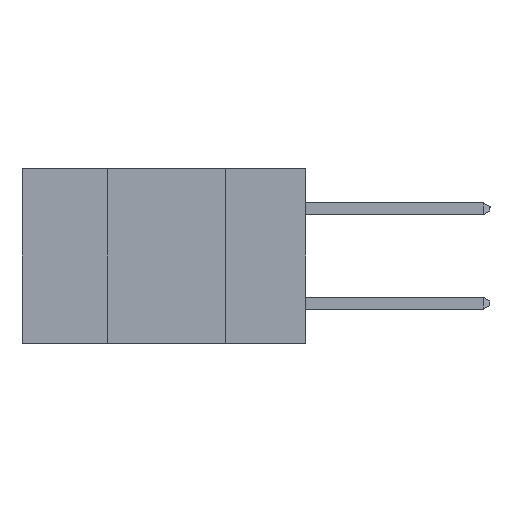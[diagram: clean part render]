
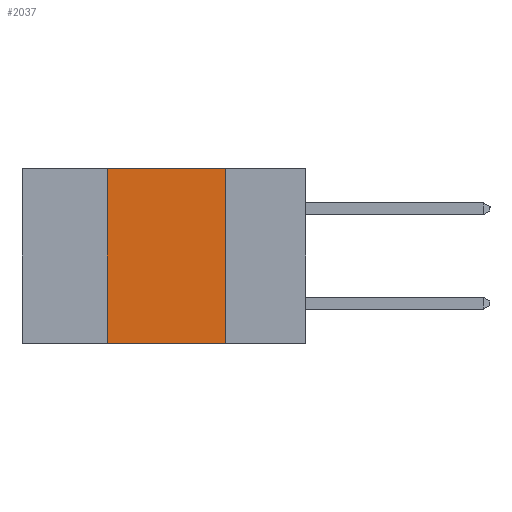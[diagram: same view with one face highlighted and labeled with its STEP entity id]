
A CAD part, left-side view. The second image highlights one B-rep face of the part: STEP entity #2037.
In plain terms, the highlighted planar face has unit normal (-1, 0, 0).
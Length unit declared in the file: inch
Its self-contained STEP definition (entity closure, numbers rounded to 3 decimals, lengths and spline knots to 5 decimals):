
#66 = EDGE_CURVE ( 'NONE', #7229, #17904, #19563, .T. ) ;
#661 = ORIENTED_EDGE ( 'NONE', *, *, #20255, .F. ) ;
#820 = CARTESIAN_POINT ( 'NONE',  ( 0., 0.6, -0.37 ) ) ;
#1248 = CARTESIAN_POINT ( 'NONE',  ( 0., 0.17, 0. ) ) ;
#1910 = ORIENTED_EDGE ( 'NONE', *, *, #20280, .F. ) ;
#2037 = ADVANCED_FACE ( 'NONE', ( #21486 ), #11666, .F. ) ;
#2146 = LINE ( 'NONE', #3776, #16999 ) ;
#2251 = LINE ( 'NONE', #17188, #3071 ) ;
#3071 = VECTOR ( 'NONE', #4003, 39.37008 ) ;
#3157 = VECTOR ( 'NONE', #4212, 39.37008 ) ;
#3263 = DIRECTION ( 'NONE',  ( 1., 0., 0. ) ) ;
#3776 = CARTESIAN_POINT ( 'NONE',  ( 0., 0.6, 0. ) ) ;
#4003 = DIRECTION ( 'NONE',  ( 0., 0., -1. ) ) ;
#4212 = DIRECTION ( 'NONE',  ( 0., -1., 0. ) ) ;
#4637 = CARTESIAN_POINT ( 'NONE',  ( 0., 0.42, -0.37 ) ) ;
#4937 = EDGE_LOOP ( 'NONE', ( #1910, #661, #10932, #7019 ) ) ;
#4977 = CARTESIAN_POINT ( 'NONE',  ( 0., 0.42, 0. ) ) ;
#6094 = VERTEX_POINT ( 'NONE', #1248 ) ;
#6374 = DIRECTION ( 'NONE',  ( 0., 0., 1. ) ) ;
#6535 = DIRECTION ( 'NONE',  ( 0., 0., -1. ) ) ;
#7019 = ORIENTED_EDGE ( 'NONE', *, *, #14820, .T. ) ;
#7229 = VERTEX_POINT ( 'NONE', #17246 ) ;
#10932 = ORIENTED_EDGE ( 'NONE', *, *, #66, .F. ) ;
#11666 = PLANE ( 'NONE',  #15181 ) ;
#12954 = VECTOR ( 'NONE', #6374, 39.37008 ) ;
#13666 = VERTEX_POINT ( 'NONE', #15384 ) ;
#14820 = EDGE_CURVE ( 'NONE', #7229, #13666, #15766, .T. ) ;
#15181 = AXIS2_PLACEMENT_3D ( 'NONE', #16675, #3263, #6535 ) ;
#15384 = CARTESIAN_POINT ( 'NONE',  ( 0., 0.17, -0.37 ) ) ;
#15766 = LINE ( 'NONE', #820, #3157 ) ;
#16675 = CARTESIAN_POINT ( 'NONE',  ( 0., 0.6, 0. ) ) ;
#16999 = VECTOR ( 'NONE', #17290, 39.37008 ) ;
#17188 = CARTESIAN_POINT ( 'NONE',  ( 0., 0.17, -0.37 ) ) ;
#17246 = CARTESIAN_POINT ( 'NONE',  ( 0., 0.42, -0.37 ) ) ;
#17290 = DIRECTION ( 'NONE',  ( 0., -1., 0. ) ) ;
#17904 = VERTEX_POINT ( 'NONE', #4977 ) ;
#19563 = LINE ( 'NONE', #4637, #12954 ) ;
#20255 = EDGE_CURVE ( 'NONE', #17904, #6094, #2146, .T. ) ;
#20280 = EDGE_CURVE ( 'NONE', #6094, #13666, #2251, .T. ) ;
#21486 = FACE_OUTER_BOUND ( 'NONE', #4937, .T. ) ;
